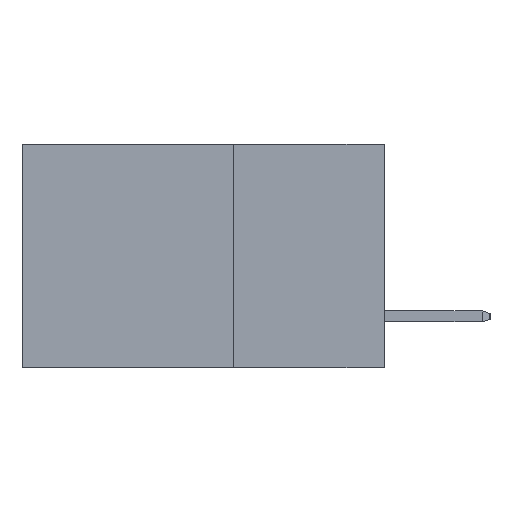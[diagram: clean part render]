
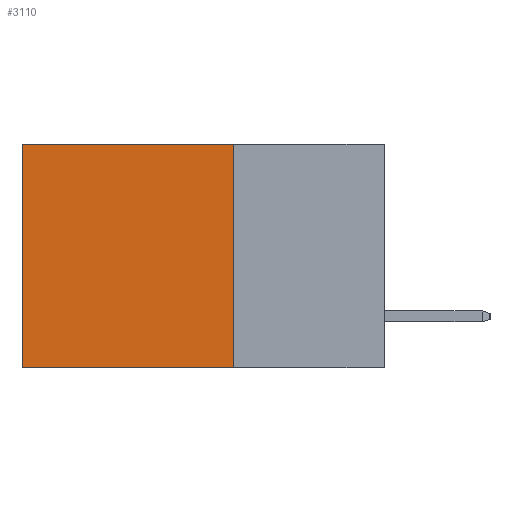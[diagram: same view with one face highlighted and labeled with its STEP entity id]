
A CAD part, left-side view. The second image highlights one B-rep face of the part: STEP entity #3110.
In plain terms, the highlighted planar face has unit normal (-1, 0, 0).
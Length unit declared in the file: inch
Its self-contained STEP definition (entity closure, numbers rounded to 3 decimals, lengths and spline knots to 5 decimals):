
#1074 = AXIS2_PLACEMENT_3D ( 'NONE', #10625, #9628, #9302 ) ;
#1680 = ORIENTED_EDGE ( 'NONE', *, *, #13510, .T. ) ;
#1813 = ORIENTED_EDGE ( 'NONE', *, *, #9729, .F. ) ;
#2131 = VECTOR ( 'NONE', #12494, 39.37008 ) ;
#2230 = VECTOR ( 'NONE', #12161, 39.37008 ) ;
#3110 = ADVANCED_FACE ( 'NONE', ( #12022 ), #9411, .F. ) ;
#4552 = VECTOR ( 'NONE', #8336, 39.37008 ) ;
#4925 = CARTESIAN_POINT ( 'NONE',  ( 0.2615, 0.25, 0. ) ) ;
#6007 = EDGE_LOOP ( 'NONE', ( #1680, #1813, #10722, #13602 ) ) ;
#6931 = CARTESIAN_POINT ( 'NONE',  ( 0.2615, 0.25, 0. ) ) ;
#8336 = DIRECTION ( 'NONE',  ( 0., 0., -1. ) ) ;
#8380 = CARTESIAN_POINT ( 'NONE',  ( 0.2615, 0.25, -0.37 ) ) ;
#8495 = DIRECTION ( 'NONE',  ( 0., 1., 0. ) ) ;
#9302 = DIRECTION ( 'NONE',  ( 0., 0., -1. ) ) ;
#9411 = PLANE ( 'NONE',  #1074 ) ;
#9628 = DIRECTION ( 'NONE',  ( 1., 0., 0. ) ) ;
#9729 = EDGE_CURVE ( 'NONE', #12324, #16327, #13786, .T. ) ;
#9951 = EDGE_CURVE ( 'NONE', #14250, #11351, #14240, .T. ) ;
#10625 = CARTESIAN_POINT ( 'NONE',  ( 0.2615, 0.25, -0.37 ) ) ;
#10679 = CARTESIAN_POINT ( 'NONE',  ( 0.2615, 0.6, -0.37 ) ) ;
#10722 = ORIENTED_EDGE ( 'NONE', *, *, #12969, .F. ) ;
#11351 = VERTEX_POINT ( 'NONE', #17800 ) ;
#12022 = FACE_OUTER_BOUND ( 'NONE', #6007, .T. ) ;
#12161 = DIRECTION ( 'NONE',  ( 0., 0., -1. ) ) ;
#12324 = VERTEX_POINT ( 'NONE', #14903 ) ;
#12494 = DIRECTION ( 'NONE',  ( 0., 1., 0. ) ) ;
#12804 = LINE ( 'NONE', #8380, #4552 ) ;
#12969 = EDGE_CURVE ( 'NONE', #14250, #12324, #12804, .T. ) ;
#13510 = EDGE_CURVE ( 'NONE', #11351, #16327, #13878, .T. ) ;
#13602 = ORIENTED_EDGE ( 'NONE', *, *, #9951, .T. ) ;
#13786 = LINE ( 'NONE', #14904, #2131 ) ;
#13878 = LINE ( 'NONE', #10679, #2230 ) ;
#14240 = LINE ( 'NONE', #6931, #17428 ) ;
#14250 = VERTEX_POINT ( 'NONE', #4925 ) ;
#14903 = CARTESIAN_POINT ( 'NONE',  ( 0.2615, 0.25, -0.37 ) ) ;
#14904 = CARTESIAN_POINT ( 'NONE',  ( 0.2615, 0.25, -0.37 ) ) ;
#16327 = VERTEX_POINT ( 'NONE', #17552 ) ;
#17428 = VECTOR ( 'NONE', #8495, 39.37008 ) ;
#17552 = CARTESIAN_POINT ( 'NONE',  ( 0.2615, 0.6, -0.37 ) ) ;
#17800 = CARTESIAN_POINT ( 'NONE',  ( 0.2615, 0.6, 0. ) ) ;
